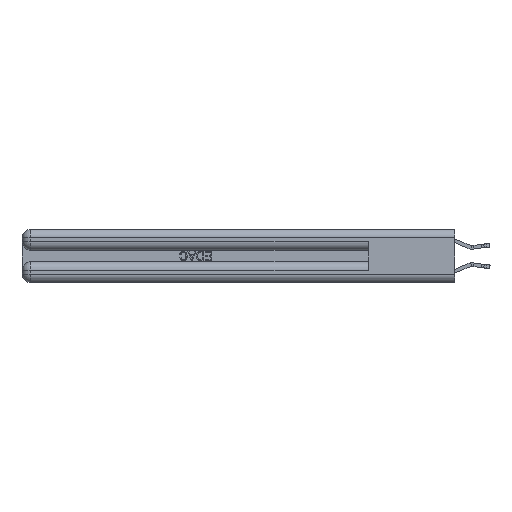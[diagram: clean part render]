
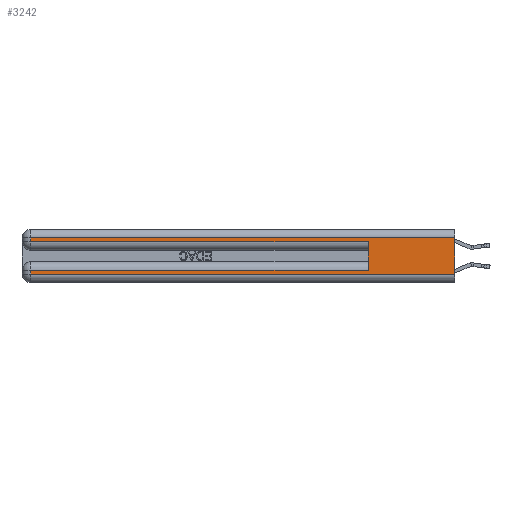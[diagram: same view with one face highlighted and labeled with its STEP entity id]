
A CAD part, left-side view. The second image highlights one B-rep face of the part: STEP entity #3242.
In plain terms, the highlighted planar face has unit normal (-1, 0, 0).
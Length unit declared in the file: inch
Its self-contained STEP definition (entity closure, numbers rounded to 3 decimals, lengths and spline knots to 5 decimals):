
#166 = LINE ( 'NONE', #19725, #18227 ) ;
#606 = CARTESIAN_POINT ( 'NONE',  ( 0., 0.6, 0.145 ) ) ;
#694 = LINE ( 'NONE', #11832, #25364 ) ;
#1425 = VERTEX_POINT ( 'NONE', #18308 ) ;
#1520 = EDGE_CURVE ( 'NONE', #28813, #10488, #694, .T. ) ;
#2078 = CARTESIAN_POINT ( 'NONE',  ( 0., 0., 0.06 ) ) ;
#2549 = CARTESIAN_POINT ( 'NONE',  ( 0., 2.94, 0.31 ) ) ;
#2551 = ORIENTED_EDGE ( 'NONE', *, *, #29032, .T. ) ;
#2600 = LINE ( 'NONE', #23880, #23364 ) ;
#2927 = CARTESIAN_POINT ( 'NONE',  ( 0., 2.94, 0.37 ) ) ;
#2967 = CARTESIAN_POINT ( 'NONE',  ( 0., 2.94, 0.085 ) ) ;
#3242 = ADVANCED_FACE ( 'NONE', ( #6360 ), #20660, .F. ) ;
#4071 = VERTEX_POINT ( 'NONE', #2078 ) ;
#4675 = VERTEX_POINT ( 'NONE', #26173 ) ;
#5978 = DIRECTION ( 'NONE',  ( 0., 0., -1. ) ) ;
#6084 = LINE ( 'NONE', #17758, #29980 ) ;
#6360 = FACE_OUTER_BOUND ( 'NONE', #10673, .T. ) ;
#7144 = LINE ( 'NONE', #18999, #19809 ) ;
#7774 = CARTESIAN_POINT ( 'NONE',  ( 0., 0., 0.37 ) ) ;
#8216 = VECTOR ( 'NONE', #12472, 39.37008 ) ;
#8265 = ORIENTED_EDGE ( 'NONE', *, *, #27289, .T. ) ;
#8975 = VERTEX_POINT ( 'NONE', #2549 ) ;
#9416 = CARTESIAN_POINT ( 'NONE',  ( 0., 0.6, 0.085 ) ) ;
#9488 = CARTESIAN_POINT ( 'NONE',  ( 0., 0., 0.31 ) ) ;
#9673 = ORIENTED_EDGE ( 'NONE', *, *, #17411, .T. ) ;
#10488 = VERTEX_POINT ( 'NONE', #2967 ) ;
#10673 = EDGE_LOOP ( 'NONE', ( #28776, #2551, #9673, #23928, #11394, #29671, #24885, #8265 ) ) ;
#11394 = ORIENTED_EDGE ( 'NONE', *, *, #14713, .F. ) ;
#11832 = CARTESIAN_POINT ( 'NONE',  ( 0., 0., 0.085 ) ) ;
#12292 = LINE ( 'NONE', #606, #28527 ) ;
#12472 = DIRECTION ( 'NONE',  ( 0., 0., -1. ) ) ;
#14308 = DIRECTION ( 'NONE',  ( 0., 1., 0. ) ) ;
#14713 = EDGE_CURVE ( 'NONE', #28813, #21553, #12292, .T. ) ;
#15810 = CARTESIAN_POINT ( 'NONE',  ( 0., 0., 0.37 ) ) ;
#17411 = EDGE_CURVE ( 'NONE', #8975, #1425, #7144, .T. ) ;
#17758 = CARTESIAN_POINT ( 'NONE',  ( 0., 0., 0.285 ) ) ;
#18227 = VECTOR ( 'NONE', #25024, 39.37008 ) ;
#18308 = CARTESIAN_POINT ( 'NONE',  ( 0., 2.94, 0.285 ) ) ;
#18999 = CARTESIAN_POINT ( 'NONE',  ( 0., 2.94, 0.37 ) ) ;
#19725 = CARTESIAN_POINT ( 'NONE',  ( 0., 0., 0.31 ) ) ;
#19809 = VECTOR ( 'NONE', #31123, 39.37008 ) ;
#20145 = LINE ( 'NONE', #7774, #8216 ) ;
#20434 = DIRECTION ( 'NONE',  ( 0., 0., -1. ) ) ;
#20660 = PLANE ( 'NONE',  #31858 ) ;
#20959 = VERTEX_POINT ( 'NONE', #9488 ) ;
#20980 = DIRECTION ( 'NONE',  ( 1., 0., 0. ) ) ;
#21057 = CARTESIAN_POINT ( 'NONE',  ( 0., 0.6, 0.285 ) ) ;
#21279 = DIRECTION ( 'NONE',  ( 0., -1., 0. ) ) ;
#21553 = VERTEX_POINT ( 'NONE', #21057 ) ;
#23364 = VECTOR ( 'NONE', #21279, 39.37008 ) ;
#23554 = VECTOR ( 'NONE', #20434, 39.37008 ) ;
#23880 = CARTESIAN_POINT ( 'NONE',  ( 0., 0., 0.06 ) ) ;
#23928 = ORIENTED_EDGE ( 'NONE', *, *, #27037, .T. ) ;
#24885 = ORIENTED_EDGE ( 'NONE', *, *, #27081, .T. ) ;
#24952 = DIRECTION ( 'NONE',  ( 0., 0., 1. ) ) ;
#25024 = DIRECTION ( 'NONE',  ( 0., 1., 0. ) ) ;
#25104 = DIRECTION ( 'NONE',  ( 0., -1., 0. ) ) ;
#25364 = VECTOR ( 'NONE', #14308, 39.37008 ) ;
#26173 = CARTESIAN_POINT ( 'NONE',  ( 0., 2.94, 0.06 ) ) ;
#27037 = EDGE_CURVE ( 'NONE', #1425, #21553, #6084, .T. ) ;
#27081 = EDGE_CURVE ( 'NONE', #10488, #4675, #30991, .T. ) ;
#27289 = EDGE_CURVE ( 'NONE', #4675, #4071, #2600, .T. ) ;
#28527 = VECTOR ( 'NONE', #24952, 39.37008 ) ;
#28776 = ORIENTED_EDGE ( 'NONE', *, *, #29600, .F. ) ;
#28813 = VERTEX_POINT ( 'NONE', #9416 ) ;
#29032 = EDGE_CURVE ( 'NONE', #20959, #8975, #166, .T. ) ;
#29600 = EDGE_CURVE ( 'NONE', #20959, #4071, #20145, .T. ) ;
#29671 = ORIENTED_EDGE ( 'NONE', *, *, #1520, .T. ) ;
#29980 = VECTOR ( 'NONE', #25104, 39.37008 ) ;
#30991 = LINE ( 'NONE', #2927, #23554 ) ;
#31123 = DIRECTION ( 'NONE',  ( 0., 0., -1. ) ) ;
#31858 = AXIS2_PLACEMENT_3D ( 'NONE', #15810, #20980, #5978 ) ;
